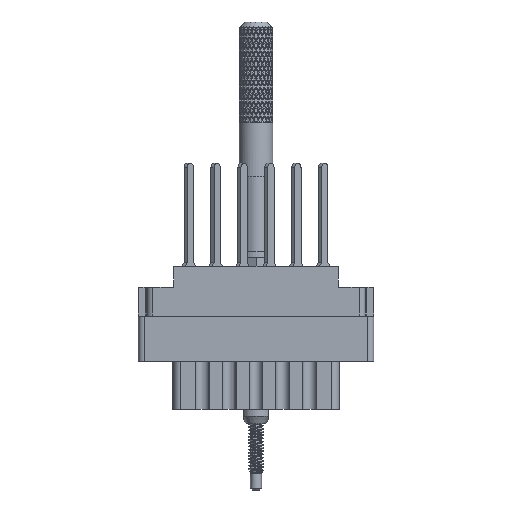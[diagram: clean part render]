
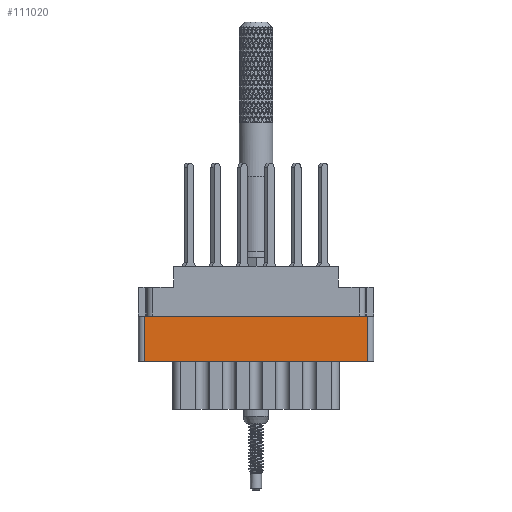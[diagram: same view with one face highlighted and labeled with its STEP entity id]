
A CAD part, front view. The second image highlights one B-rep face of the part: STEP entity #111020.
In plain terms, the highlighted planar face has unit normal (0, -1, 0).
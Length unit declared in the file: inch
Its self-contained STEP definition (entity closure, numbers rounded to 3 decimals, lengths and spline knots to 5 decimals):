
#14149 = ORIENTED_EDGE ( 'NONE', *, *, #54313, .F. ) ;
#18570 = DIRECTION ( 'NONE',  ( 0., 0., 1. ) ) ;
#32383 = CARTESIAN_POINT ( 'NONE',  ( 0.624, -0.343, -0.529 ) ) ;
#35769 = VERTEX_POINT ( 'NONE', #65772 ) ;
#41328 = LINE ( 'NONE', #156146, #83731 ) ;
#48991 = LINE ( 'NONE', #32383, #50495 ) ;
#50495 = VECTOR ( 'NONE', #132444, 39.37008 ) ;
#52213 = VERTEX_POINT ( 'NONE', #98299 ) ;
#54313 = EDGE_CURVE ( 'NONE', #52213, #149166, #41328, .T. ) ;
#55593 = EDGE_CURVE ( 'NONE', #168559, #149166, #145476, .T. ) ;
#58353 = CARTESIAN_POINT ( 'NONE',  ( -0.624, -0.343, -0.798 ) ) ;
#63510 = EDGE_CURVE ( 'NONE', #35769, #52213, #91422, .T. ) ;
#64932 = PLANE ( 'NONE',  #144286 ) ;
#65772 = CARTESIAN_POINT ( 'NONE',  ( -0.624, -0.343, -0.529 ) ) ;
#73251 = CARTESIAN_POINT ( 'NONE',  ( 0.624, -0.343, -0.798 ) ) ;
#76940 = CARTESIAN_POINT ( 'NONE',  ( 0.624, -0.343, -0.529 ) ) ;
#83731 = VECTOR ( 'NONE', #96952, 39.37008 ) ;
#91422 = LINE ( 'NONE', #58353, #122593 ) ;
#96952 = DIRECTION ( 'NONE',  ( 1., 0., 0. ) ) ;
#98299 = CARTESIAN_POINT ( 'NONE',  ( -0.624, -0.343, -0.277 ) ) ;
#111020 = ADVANCED_FACE ( 'NONE', ( #163135 ), #64932, .T. ) ;
#122369 = DIRECTION ( 'NONE',  ( 0., 0., -1. ) ) ;
#122593 = VECTOR ( 'NONE', #134068, 39.37008 ) ;
#129455 = ORIENTED_EDGE ( 'NONE', *, *, #136338, .F. ) ;
#132444 = DIRECTION ( 'NONE',  ( -1., 0., 0. ) ) ;
#134068 = DIRECTION ( 'NONE',  ( 0., 0., 1. ) ) ;
#136338 = EDGE_CURVE ( 'NONE', #168559, #35769, #48991, .T. ) ;
#137456 = ORIENTED_EDGE ( 'NONE', *, *, #55593, .T. ) ;
#138101 = DIRECTION ( 'NONE',  ( 0., -1., 0. ) ) ;
#144286 = AXIS2_PLACEMENT_3D ( 'NONE', #151059, #138101, #122369 ) ;
#145476 = LINE ( 'NONE', #73251, #181401 ) ;
#149166 = VERTEX_POINT ( 'NONE', #167702 ) ;
#151059 = CARTESIAN_POINT ( 'NONE',  ( -0.624, -0.343, -0.798 ) ) ;
#154585 = ORIENTED_EDGE ( 'NONE', *, *, #63510, .F. ) ;
#156146 = CARTESIAN_POINT ( 'NONE',  ( -0.656, -0.343, -0.277 ) ) ;
#157680 = EDGE_LOOP ( 'NONE', ( #154585, #129455, #137456, #14149 ) ) ;
#163135 = FACE_OUTER_BOUND ( 'NONE', #157680, .T. ) ;
#167702 = CARTESIAN_POINT ( 'NONE',  ( 0.624, -0.343, -0.277 ) ) ;
#168559 = VERTEX_POINT ( 'NONE', #76940 ) ;
#181401 = VECTOR ( 'NONE', #18570, 39.37008 ) ;
